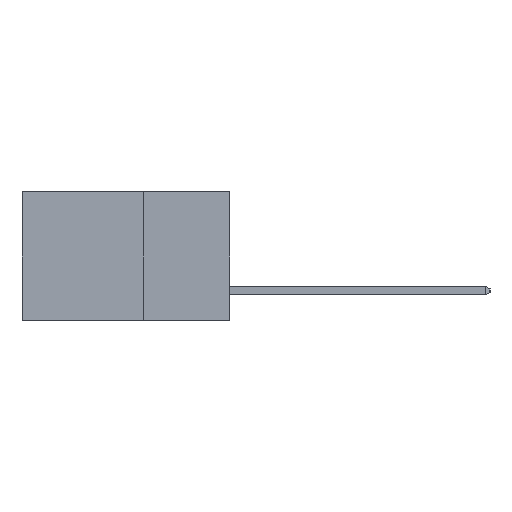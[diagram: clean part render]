
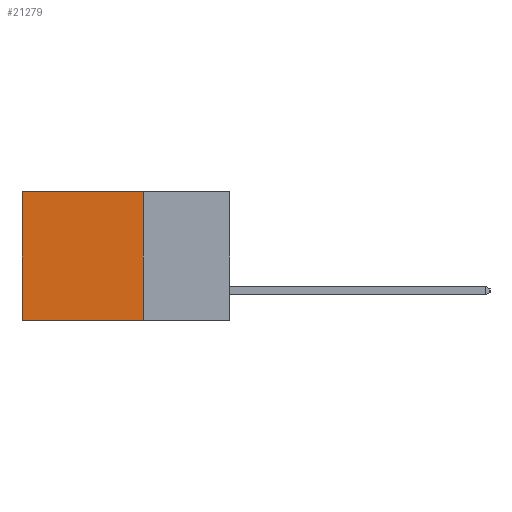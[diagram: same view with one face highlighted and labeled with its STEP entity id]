
A CAD part, left-side view. The second image highlights one B-rep face of the part: STEP entity #21279.
In plain terms, the highlighted planar face has unit normal (-1, 0, 0).
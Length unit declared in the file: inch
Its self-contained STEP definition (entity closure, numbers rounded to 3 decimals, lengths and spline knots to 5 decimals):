
#255 = PLANE ( 'NONE',  #21056 ) ;
#655 = EDGE_CURVE ( 'NONE', #21212, #1089, #22259, .T. ) ;
#1089 = VERTEX_POINT ( 'NONE', #9178 ) ;
#1153 = LINE ( 'NONE', #4212, #5430 ) ;
#1567 = FACE_OUTER_BOUND ( 'NONE', #12278, .T. ) ;
#1871 = ORIENTED_EDGE ( 'NONE', *, *, #5922, .F. ) ;
#2072 = DIRECTION ( 'NONE',  ( 1., 0., 0. ) ) ;
#3351 = DIRECTION ( 'NONE',  ( 0., 0., -1. ) ) ;
#3465 = ORIENTED_EDGE ( 'NONE', *, *, #655, .F. ) ;
#3835 = DIRECTION ( 'NONE',  ( 0., 0., -1. ) ) ;
#4106 = DIRECTION ( 'NONE',  ( 0., 1., 0. ) ) ;
#4212 = CARTESIAN_POINT ( 'NONE',  ( 0.2615, 0.25, 0. ) ) ;
#4242 = VECTOR ( 'NONE', #3835, 39.37008 ) ;
#5326 = CARTESIAN_POINT ( 'NONE',  ( 0.2615, 0.25, -0.37 ) ) ;
#5430 = VECTOR ( 'NONE', #4106, 39.37008 ) ;
#5699 = VECTOR ( 'NONE', #3351, 39.37008 ) ;
#5922 = EDGE_CURVE ( 'NONE', #14451, #21212, #14433, .T. ) ;
#6539 = VERTEX_POINT ( 'NONE', #18348 ) ;
#7537 = ORIENTED_EDGE ( 'NONE', *, *, #19009, .T. ) ;
#9178 = CARTESIAN_POINT ( 'NONE',  ( 0.2615, 0.6, -0.37 ) ) ;
#12278 = EDGE_LOOP ( 'NONE', ( #7537, #3465, #1871, #15785 ) ) ;
#12525 = EDGE_CURVE ( 'NONE', #14451, #6539, #1153, .T. ) ;
#13428 = CARTESIAN_POINT ( 'NONE',  ( 0.2615, 0.25, -0.37 ) ) ;
#13559 = VECTOR ( 'NONE', #15412, 39.37008 ) ;
#14433 = LINE ( 'NONE', #5326, #4242 ) ;
#14451 = VERTEX_POINT ( 'NONE', #18696 ) ;
#14511 = CARTESIAN_POINT ( 'NONE',  ( 0.2615, 0.25, -0.37 ) ) ;
#14755 = DIRECTION ( 'NONE',  ( 0., 0., -1. ) ) ;
#15412 = DIRECTION ( 'NONE',  ( 0., 1., 0. ) ) ;
#15785 = ORIENTED_EDGE ( 'NONE', *, *, #12525, .T. ) ;
#18348 = CARTESIAN_POINT ( 'NONE',  ( 0.2615, 0.6, 0. ) ) ;
#18696 = CARTESIAN_POINT ( 'NONE',  ( 0.2615, 0.25, 0. ) ) ;
#19009 = EDGE_CURVE ( 'NONE', #6539, #1089, #19935, .T. ) ;
#19935 = LINE ( 'NONE', #21224, #5699 ) ;
#21056 = AXIS2_PLACEMENT_3D ( 'NONE', #21671, #2072, #14755 ) ;
#21212 = VERTEX_POINT ( 'NONE', #14511 ) ;
#21224 = CARTESIAN_POINT ( 'NONE',  ( 0.2615, 0.6, -0.37 ) ) ;
#21279 = ADVANCED_FACE ( 'NONE', ( #1567 ), #255, .F. ) ;
#21671 = CARTESIAN_POINT ( 'NONE',  ( 0.2615, 0.25, -0.37 ) ) ;
#22259 = LINE ( 'NONE', #13428, #13559 ) ;
